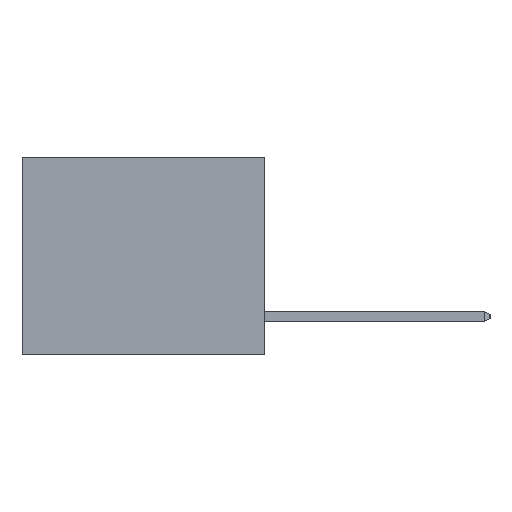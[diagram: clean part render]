
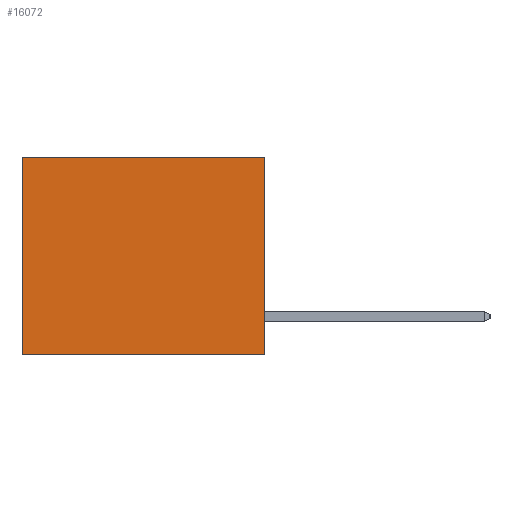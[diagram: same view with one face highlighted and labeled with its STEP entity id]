
A CAD part, left-side view. The second image highlights one B-rep face of the part: STEP entity #16072.
In plain terms, the highlighted planar face has unit normal (-1, 0, 0).
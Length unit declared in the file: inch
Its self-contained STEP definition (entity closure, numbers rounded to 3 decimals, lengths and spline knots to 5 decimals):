
#1030 = ORIENTED_EDGE ( 'NONE', *, *, #11014, .F. ) ;
#1220 = AXIS2_PLACEMENT_3D ( 'NONE', #24118, #9546, #11586 ) ;
#1747 = ORIENTED_EDGE ( 'NONE', *, *, #15468, .T. ) ;
#2648 = CARTESIAN_POINT ( 'NONE',  ( 0.3165, 0.6, -0.49 ) ) ;
#2841 = VECTOR ( 'NONE', #27150, 39.37008 ) ;
#3153 = PLANE ( 'NONE',  #1220 ) ;
#5235 = DIRECTION ( 'NONE',  ( 0., 0., -1. ) ) ;
#5654 = CARTESIAN_POINT ( 'NONE',  ( 0.3165, 0., -0.49 ) ) ;
#6500 = LINE ( 'NONE', #21756, #22664 ) ;
#7839 = LINE ( 'NONE', #10286, #2841 ) ;
#9147 = CARTESIAN_POINT ( 'NONE',  ( 0.3165, 0., 0. ) ) ;
#9546 = DIRECTION ( 'NONE',  ( 1., 0., 0. ) ) ;
#10086 = VECTOR ( 'NONE', #21972, 39.37008 ) ;
#10286 = CARTESIAN_POINT ( 'NONE',  ( 0.3165, 0.6, -0.49 ) ) ;
#11014 = EDGE_CURVE ( 'NONE', #16554, #24241, #11710, .T. ) ;
#11586 = DIRECTION ( 'NONE',  ( 0., 0., -1. ) ) ;
#11710 = LINE ( 'NONE', #26886, #14672 ) ;
#12031 = ORIENTED_EDGE ( 'NONE', *, *, #21287, .T. ) ;
#12235 = DIRECTION ( 'NONE',  ( 0., 1., 0. ) ) ;
#13490 = CARTESIAN_POINT ( 'NONE',  ( 0.3165, 0., 0. ) ) ;
#14672 = VECTOR ( 'NONE', #12235, 39.37008 ) ;
#15233 = EDGE_CURVE ( 'NONE', #20621, #16554, #6500, .T. ) ;
#15468 = EDGE_CURVE ( 'NONE', #20621, #23956, #15688, .T. ) ;
#15688 = LINE ( 'NONE', #13490, #10086 ) ;
#16072 = ADVANCED_FACE ( 'NONE', ( #19276 ), #3153, .F. ) ;
#16554 = VERTEX_POINT ( 'NONE', #5654 ) ;
#18361 = EDGE_LOOP ( 'NONE', ( #12031, #1030, #20355, #1747 ) ) ;
#19197 = CARTESIAN_POINT ( 'NONE',  ( 0.3165, 0.6, 0. ) ) ;
#19276 = FACE_OUTER_BOUND ( 'NONE', #18361, .T. ) ;
#20355 = ORIENTED_EDGE ( 'NONE', *, *, #15233, .F. ) ;
#20621 = VERTEX_POINT ( 'NONE', #9147 ) ;
#21287 = EDGE_CURVE ( 'NONE', #23956, #24241, #7839, .T. ) ;
#21756 = CARTESIAN_POINT ( 'NONE',  ( 0.3165, 0., -0.49 ) ) ;
#21972 = DIRECTION ( 'NONE',  ( 0., 1., 0. ) ) ;
#22664 = VECTOR ( 'NONE', #5235, 39.37008 ) ;
#23956 = VERTEX_POINT ( 'NONE', #19197 ) ;
#24118 = CARTESIAN_POINT ( 'NONE',  ( 0.3165, 0., -0.49 ) ) ;
#24241 = VERTEX_POINT ( 'NONE', #2648 ) ;
#26886 = CARTESIAN_POINT ( 'NONE',  ( 0.3165, 0., -0.49 ) ) ;
#27150 = DIRECTION ( 'NONE',  ( 0., 0., -1. ) ) ;
